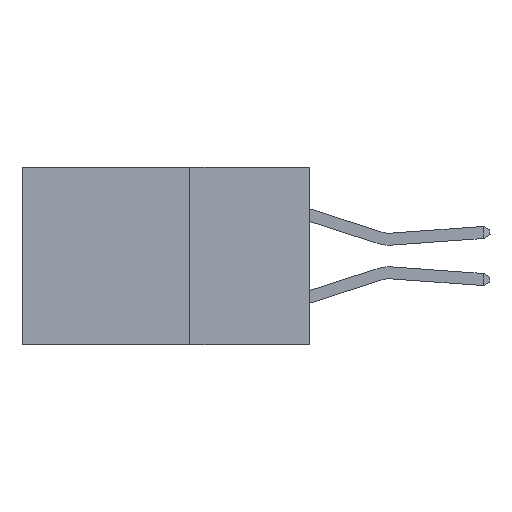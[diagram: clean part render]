
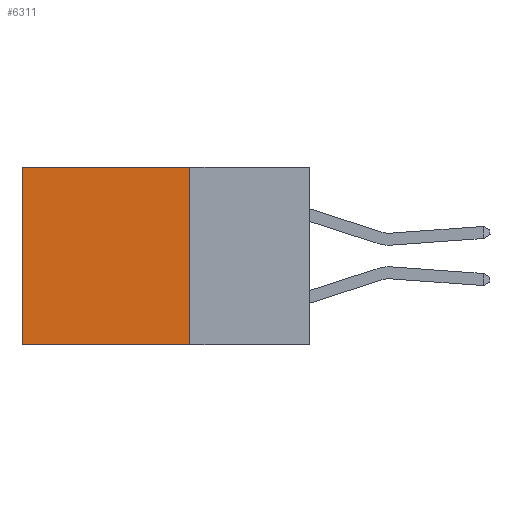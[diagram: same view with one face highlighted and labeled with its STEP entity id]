
A CAD part, left-side view. The second image highlights one B-rep face of the part: STEP entity #6311.
In plain terms, the highlighted planar face has unit normal (-1, 0, 0).
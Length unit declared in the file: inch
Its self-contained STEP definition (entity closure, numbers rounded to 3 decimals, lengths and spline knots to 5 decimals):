
#71 = VECTOR ( 'NONE', #13452, 39.37008 ) ;
#442 = LINE ( 'NONE', #12598, #71 ) ;
#846 = EDGE_CURVE ( 'NONE', #6414, #1092, #442, .T. ) ;
#1092 = VERTEX_POINT ( 'NONE', #12270 ) ;
#1506 = LINE ( 'NONE', #7229, #10533 ) ;
#2980 = FACE_OUTER_BOUND ( 'NONE', #5539, .T. ) ;
#3165 = DIRECTION ( 'NONE',  ( 0., 0., -1. ) ) ;
#3292 = CARTESIAN_POINT ( 'NONE',  ( 0.2615, 0.25, -0.37 ) ) ;
#3345 = CARTESIAN_POINT ( 'NONE',  ( 0.2615, 0.25, -0.37 ) ) ;
#3802 = ORIENTED_EDGE ( 'NONE', *, *, #846, .F. ) ;
#4039 = EDGE_CURVE ( 'NONE', #12519, #9263, #1506, .T. ) ;
#4667 = LINE ( 'NONE', #3345, #5046 ) ;
#5046 = VECTOR ( 'NONE', #3165, 39.37008 ) ;
#5539 = EDGE_LOOP ( 'NONE', ( #7102, #3802, #6411, #6199 ) ) ;
#6199 = ORIENTED_EDGE ( 'NONE', *, *, #4039, .T. ) ;
#6311 = ADVANCED_FACE ( 'NONE', ( #2980 ), #10171, .F. ) ;
#6411 = ORIENTED_EDGE ( 'NONE', *, *, #14229, .F. ) ;
#6414 = VERTEX_POINT ( 'NONE', #3292 ) ;
#6914 = DIRECTION ( 'NONE',  ( 0., 1., 0. ) ) ;
#7102 = ORIENTED_EDGE ( 'NONE', *, *, #10670, .T. ) ;
#7147 = VECTOR ( 'NONE', #11239, 39.37008 ) ;
#7229 = CARTESIAN_POINT ( 'NONE',  ( 0.2615, 0.25, 0. ) ) ;
#9263 = VERTEX_POINT ( 'NONE', #9970 ) ;
#9964 = CARTESIAN_POINT ( 'NONE',  ( 0.2615, 0.25, 0. ) ) ;
#9970 = CARTESIAN_POINT ( 'NONE',  ( 0.2615, 0.6, 0. ) ) ;
#9981 = DIRECTION ( 'NONE',  ( 1., 0., 0. ) ) ;
#9994 = DIRECTION ( 'NONE',  ( 0., 0., -1. ) ) ;
#10103 = LINE ( 'NONE', #11463, #7147 ) ;
#10171 = PLANE ( 'NONE',  #10695 ) ;
#10278 = CARTESIAN_POINT ( 'NONE',  ( 0.2615, 0.25, -0.37 ) ) ;
#10533 = VECTOR ( 'NONE', #6914, 39.37008 ) ;
#10670 = EDGE_CURVE ( 'NONE', #9263, #1092, #10103, .T. ) ;
#10695 = AXIS2_PLACEMENT_3D ( 'NONE', #10278, #9981, #9994 ) ;
#11239 = DIRECTION ( 'NONE',  ( 0., 0., -1. ) ) ;
#11463 = CARTESIAN_POINT ( 'NONE',  ( 0.2615, 0.6, -0.37 ) ) ;
#12270 = CARTESIAN_POINT ( 'NONE',  ( 0.2615, 0.6, -0.37 ) ) ;
#12519 = VERTEX_POINT ( 'NONE', #9964 ) ;
#12598 = CARTESIAN_POINT ( 'NONE',  ( 0.2615, 0.25, -0.37 ) ) ;
#13452 = DIRECTION ( 'NONE',  ( 0., 1., 0. ) ) ;
#14229 = EDGE_CURVE ( 'NONE', #12519, #6414, #4667, .T. ) ;
